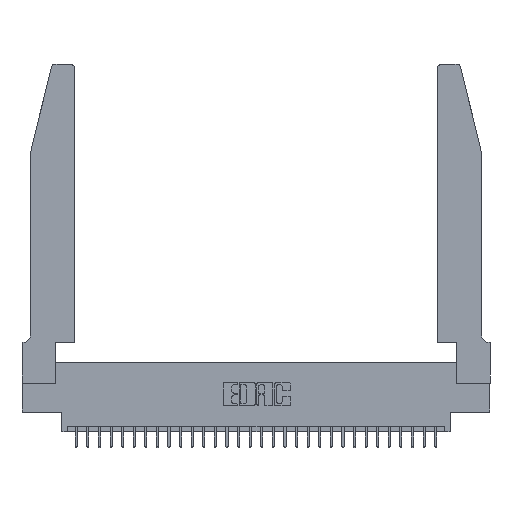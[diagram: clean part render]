
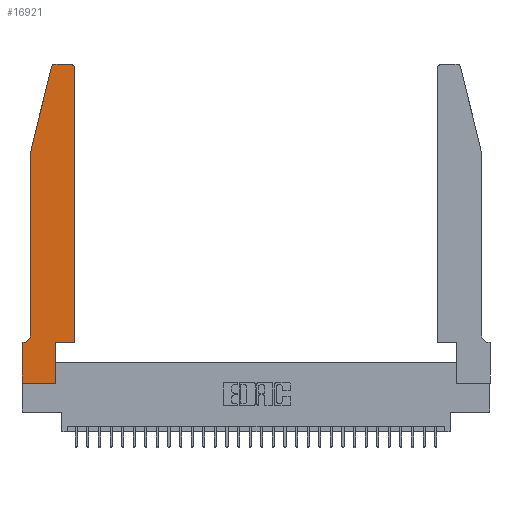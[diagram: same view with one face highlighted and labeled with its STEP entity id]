
A CAD part, top view. The second image highlights one B-rep face of the part: STEP entity #16921.
In plain terms, the highlighted planar face has unit normal (0, 0, 1).
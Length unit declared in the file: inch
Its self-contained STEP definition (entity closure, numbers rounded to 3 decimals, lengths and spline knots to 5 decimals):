
#396 = LINE ( 'NONE', #29360, #30077 ) ;
#534 = CARTESIAN_POINT ( 'NONE',  ( 0.0055, 0.42, 0.37 ) ) ;
#597 = VECTOR ( 'NONE', #9909, 39.37008 ) ;
#685 = LINE ( 'NONE', #24577, #27600 ) ;
#1041 = EDGE_CURVE ( 'NONE', #1140, #13848, #14311, .T. ) ;
#1140 = VERTEX_POINT ( 'NONE', #26242 ) ;
#1306 = CARTESIAN_POINT ( 'NONE',  ( 0., 0., 0.37 ) ) ;
#1455 = EDGE_CURVE ( 'NONE', #17039, #10153, #9606, .T. ) ;
#1561 = EDGE_CURVE ( 'NONE', #14669, #27868, #396, .T. ) ;
#1674 = ORIENTED_EDGE ( 'NONE', *, *, #9669, .T. ) ;
#2680 = EDGE_CURVE ( 'NONE', #27868, #26591, #11302, .T. ) ;
#2836 = DIRECTION ( 'NONE',  ( 0., 0., 1. ) ) ;
#3191 = AXIS2_PLACEMENT_3D ( 'NONE', #20294, #2836, #15380 ) ;
#3244 = VECTOR ( 'NONE', #30436, 39.37008 ) ;
#3476 = VERTEX_POINT ( 'NONE', #1306 ) ;
#3619 = DIRECTION ( 'NONE',  ( 1., 0., 0. ) ) ;
#3970 = DIRECTION ( 'NONE',  ( 1., 0., 0. ) ) ;
#4250 = VERTEX_POINT ( 'NONE', #23275 ) ;
#4255 = DIRECTION ( 'NONE',  ( 1., 0., 0. ) ) ;
#4656 = CARTESIAN_POINT ( 'NONE',  ( 0.4505, 2.72, 0.37 ) ) ;
#4662 = AXIS2_PLACEMENT_3D ( 'NONE', #16367, #26060, #4255 ) ;
#4998 = DIRECTION ( 'NONE',  ( -1., 0., 0. ) ) ;
#5146 = ORIENTED_EDGE ( 'NONE', *, *, #2680, .T. ) ;
#5175 = DIRECTION ( 'NONE',  ( 1., 0., 0. ) ) ;
#5274 = EDGE_CURVE ( 'NONE', #10153, #26257, #7796, .T. ) ;
#5544 = DIRECTION ( 'NONE',  ( 0., 1., 0. ) ) ;
#6697 = LINE ( 'NONE', #30739, #3244 ) ;
#7555 = DIRECTION ( 'NONE',  ( 0., 1., 0. ) ) ;
#7556 = VERTEX_POINT ( 'NONE', #28472 ) ;
#7685 = EDGE_CURVE ( 'NONE', #7556, #3476, #29259, .T. ) ;
#7796 = CIRCLE ( 'NONE', #27107, 0.07 ) ;
#8209 = VECTOR ( 'NONE', #14308, 39.37008 ) ;
#8494 = CARTESIAN_POINT ( 'NONE',  ( 0.0755, 0.42, 0.37 ) ) ;
#8576 = CARTESIAN_POINT ( 'NONE',  ( 0.4505, 0.35, 0.37 ) ) ;
#8769 = EDGE_CURVE ( 'NONE', #26591, #1140, #26850, .T. ) ;
#8972 = LINE ( 'NONE', #16171, #31253 ) ;
#9154 = CARTESIAN_POINT ( 'NONE',  ( 0.0755, 2., 0.37 ) ) ;
#9201 = ORIENTED_EDGE ( 'NONE', *, *, #11908, .T. ) ;
#9606 = LINE ( 'NONE', #15038, #597 ) ;
#9669 = EDGE_CURVE ( 'NONE', #4250, #17596, #29253, .T. ) ;
#9909 = DIRECTION ( 'NONE',  ( 0., -1., 0. ) ) ;
#10144 = ORIENTED_EDGE ( 'NONE', *, *, #7685, .T. ) ;
#10153 = VERTEX_POINT ( 'NONE', #8494 ) ;
#10358 = CARTESIAN_POINT ( 'NONE',  ( 0.4505, 0.35, 0.37 ) ) ;
#10466 = ORIENTED_EDGE ( 'NONE', *, *, #1455, .T. ) ;
#11119 = ORIENTED_EDGE ( 'NONE', *, *, #1041, .T. ) ;
#11281 = CARTESIAN_POINT ( 'NONE',  ( 0.25487, 2.72718, 0.37 ) ) ;
#11302 = CIRCLE ( 'NONE', #3191, 0.03 ) ;
#11707 = EDGE_LOOP ( 'NONE', ( #19100, #11119, #30489, #10466, #17037, #20085, #10144, #9201, #1674, #11790, #12070, #5146 ) ) ;
#11790 = ORIENTED_EDGE ( 'NONE', *, *, #16661, .T. ) ;
#11908 = EDGE_CURVE ( 'NONE', #3476, #4250, #685, .T. ) ;
#12064 = CARTESIAN_POINT ( 'NONE',  ( 0., 0., 0.37 ) ) ;
#12070 = ORIENTED_EDGE ( 'NONE', *, *, #1561, .T. ) ;
#12235 = CARTESIAN_POINT ( 'NONE',  ( 0.4205, 2.75, 0.37 ) ) ;
#12374 = CARTESIAN_POINT ( 'NONE',  ( 0.2605, 2.75, 0.37 ) ) ;
#13848 = VERTEX_POINT ( 'NONE', #11281 ) ;
#14308 = DIRECTION ( 'NONE',  ( 0., -1., 0. ) ) ;
#14311 = CIRCLE ( 'NONE', #4662, 0.03 ) ;
#14669 = VERTEX_POINT ( 'NONE', #10358 ) ;
#15031 = EDGE_CURVE ( 'NONE', #13848, #17039, #6697, .T. ) ;
#15038 = CARTESIAN_POINT ( 'NONE',  ( 0.0755, 2., 0.37 ) ) ;
#15380 = DIRECTION ( 'NONE',  ( 1., 0., 0. ) ) ;
#15538 = VECTOR ( 'NONE', #20126, 39.37008 ) ;
#16021 = DIRECTION ( 'NONE',  ( -1., 0., 0. ) ) ;
#16171 = CARTESIAN_POINT ( 'NONE',  ( 0.0755, 0.35, 0.37 ) ) ;
#16367 = CARTESIAN_POINT ( 'NONE',  ( 0.284, 2.72, 0.37 ) ) ;
#16598 = CARTESIAN_POINT ( 'NONE',  ( 0.0055, 0.35, 0.37 ) ) ;
#16661 = EDGE_CURVE ( 'NONE', #17596, #14669, #21454, .T. ) ;
#16921 = ADVANCED_FACE ( 'NONE', ( #17922 ), #27163, .T. ) ;
#17037 = ORIENTED_EDGE ( 'NONE', *, *, #5274, .T. ) ;
#17039 = VERTEX_POINT ( 'NONE', #9154 ) ;
#17596 = VERTEX_POINT ( 'NONE', #28943 ) ;
#17922 = FACE_OUTER_BOUND ( 'NONE', #11707, .T. ) ;
#19100 = ORIENTED_EDGE ( 'NONE', *, *, #8769, .T. ) ;
#19567 = VECTOR ( 'NONE', #3970, 39.37008 ) ;
#19975 = CARTESIAN_POINT ( 'NONE',  ( 0.2865, 0.35, 0.37 ) ) ;
#20085 = ORIENTED_EDGE ( 'NONE', *, *, #28579, .T. ) ;
#20126 = DIRECTION ( 'NONE',  ( -1., 0., 0. ) ) ;
#20294 = CARTESIAN_POINT ( 'NONE',  ( 0.4205, 2.72, 0.37 ) ) ;
#20458 = CARTESIAN_POINT ( 'NONE',  ( 0., 0.35, 0.37 ) ) ;
#21454 = LINE ( 'NONE', #8576, #19567 ) ;
#23275 = CARTESIAN_POINT ( 'NONE',  ( 0.2865, 0., 0.37 ) ) ;
#24577 = CARTESIAN_POINT ( 'NONE',  ( 0., 0., 0.37 ) ) ;
#26060 = DIRECTION ( 'NONE',  ( 0., 0., 1. ) ) ;
#26242 = CARTESIAN_POINT ( 'NONE',  ( 0.284, 2.75, 0.37 ) ) ;
#26257 = VERTEX_POINT ( 'NONE', #16598 ) ;
#26591 = VERTEX_POINT ( 'NONE', #12235 ) ;
#26850 = LINE ( 'NONE', #12374, #15538 ) ;
#27107 = AXIS2_PLACEMENT_3D ( 'NONE', #534, #29181, #4998 ) ;
#27163 = PLANE ( 'NONE',  #27732 ) ;
#27600 = VECTOR ( 'NONE', #5175, 39.37008 ) ;
#27732 = AXIS2_PLACEMENT_3D ( 'NONE', #20458, #27785, #3619 ) ;
#27785 = DIRECTION ( 'NONE',  ( 0., 0., 1. ) ) ;
#27868 = VERTEX_POINT ( 'NONE', #4656 ) ;
#28472 = CARTESIAN_POINT ( 'NONE',  ( 0., 0.35, 0.37 ) ) ;
#28579 = EDGE_CURVE ( 'NONE', #26257, #7556, #8972, .T. ) ;
#28943 = CARTESIAN_POINT ( 'NONE',  ( 0.2865, 0.35, 0.37 ) ) ;
#29181 = DIRECTION ( 'NONE',  ( 0., 0., -1. ) ) ;
#29253 = LINE ( 'NONE', #19975, #30894 ) ;
#29259 = LINE ( 'NONE', #12064, #8209 ) ;
#29360 = CARTESIAN_POINT ( 'NONE',  ( 0.4505, 0.35, 0.37 ) ) ;
#30077 = VECTOR ( 'NONE', #7555, 39.37008 ) ;
#30436 = DIRECTION ( 'NONE',  ( -0.239, -0.971, 0. ) ) ;
#30489 = ORIENTED_EDGE ( 'NONE', *, *, #15031, .T. ) ;
#30739 = CARTESIAN_POINT ( 'NONE',  ( 0.0755, 2., 0.37 ) ) ;
#30894 = VECTOR ( 'NONE', #5544, 39.37008 ) ;
#31253 = VECTOR ( 'NONE', #16021, 39.37008 ) ;
